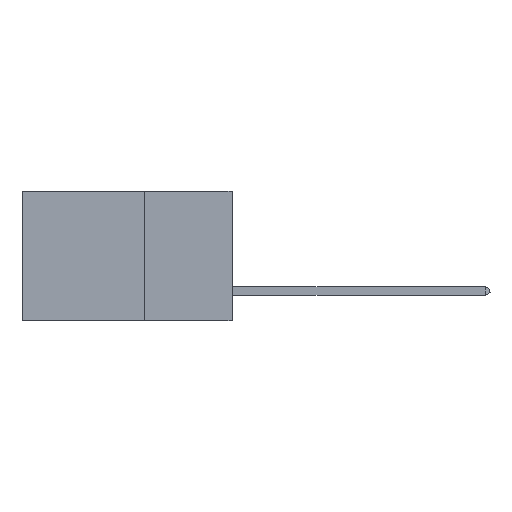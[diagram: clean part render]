
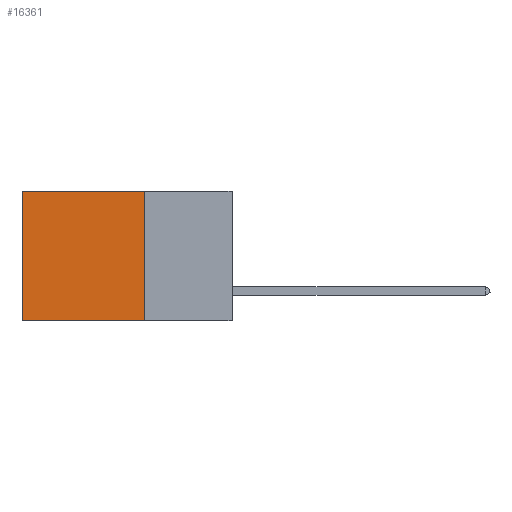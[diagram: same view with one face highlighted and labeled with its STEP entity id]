
A CAD part, left-side view. The second image highlights one B-rep face of the part: STEP entity #16361.
In plain terms, the highlighted planar face has unit normal (-1, 0, 0).
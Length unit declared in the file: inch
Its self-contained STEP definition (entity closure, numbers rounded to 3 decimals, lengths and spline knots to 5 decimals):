
#1655 = EDGE_LOOP ( 'NONE', ( #27776, #11221, #21335, #10406 ) ) ;
#3006 = VERTEX_POINT ( 'NONE', #31221 ) ;
#4205 = LINE ( 'NONE', #17229, #16119 ) ;
#4326 = LINE ( 'NONE', #5496, #10497 ) ;
#5043 = CARTESIAN_POINT ( 'NONE',  ( 0.2875, 0.25, 0. ) ) ;
#5496 = CARTESIAN_POINT ( 'NONE',  ( 0.2875, 0.25, 0. ) ) ;
#5628 = EDGE_CURVE ( 'NONE', #12628, #7341, #4205, .T. ) ;
#7341 = VERTEX_POINT ( 'NONE', #9530 ) ;
#7800 = DIRECTION ( 'NONE',  ( 0., 0., -1. ) ) ;
#9530 = CARTESIAN_POINT ( 'NONE',  ( 0.2875, 0.6, -0.37 ) ) ;
#9923 = CARTESIAN_POINT ( 'NONE',  ( 0.2875, 0.6, 0. ) ) ;
#10406 = ORIENTED_EDGE ( 'NONE', *, *, #24527, .T. ) ;
#10497 = VECTOR ( 'NONE', #31381, 39.37008 ) ;
#11221 = ORIENTED_EDGE ( 'NONE', *, *, #28537, .F. ) ;
#12135 = VECTOR ( 'NONE', #25882, 39.37008 ) ;
#12628 = VERTEX_POINT ( 'NONE', #9923 ) ;
#13090 = DIRECTION ( 'NONE',  ( 1., 0., 0. ) ) ;
#16119 = VECTOR ( 'NONE', #28268, 39.37008 ) ;
#16177 = LINE ( 'NONE', #26999, #20704 ) ;
#16361 = ADVANCED_FACE ( 'NONE', ( #22333 ), #20806, .F. ) ;
#17229 = CARTESIAN_POINT ( 'NONE',  ( 0.2875, 0.6, 0. ) ) ;
#17569 = AXIS2_PLACEMENT_3D ( 'NONE', #5043, #13090, #7800 ) ;
#20704 = VECTOR ( 'NONE', #32283, 39.37008 ) ;
#20806 = PLANE ( 'NONE',  #17569 ) ;
#20807 = LINE ( 'NONE', #25993, #12135 ) ;
#21335 = ORIENTED_EDGE ( 'NONE', *, *, #29887, .F. ) ;
#22022 = CARTESIAN_POINT ( 'NONE',  ( 0.2875, 0.25, 0. ) ) ;
#22333 = FACE_OUTER_BOUND ( 'NONE', #1655, .T. ) ;
#24527 = EDGE_CURVE ( 'NONE', #29879, #12628, #4326, .T. ) ;
#25882 = DIRECTION ( 'NONE',  ( 0., 1., 0. ) ) ;
#25993 = CARTESIAN_POINT ( 'NONE',  ( 0.2875, 0.25, -0.37 ) ) ;
#26999 = CARTESIAN_POINT ( 'NONE',  ( 0.2875, 0.25, 0. ) ) ;
#27776 = ORIENTED_EDGE ( 'NONE', *, *, #5628, .T. ) ;
#28268 = DIRECTION ( 'NONE',  ( 0., 0., -1. ) ) ;
#28537 = EDGE_CURVE ( 'NONE', #3006, #7341, #20807, .T. ) ;
#29879 = VERTEX_POINT ( 'NONE', #22022 ) ;
#29887 = EDGE_CURVE ( 'NONE', #29879, #3006, #16177, .T. ) ;
#31221 = CARTESIAN_POINT ( 'NONE',  ( 0.2875, 0.25, -0.37 ) ) ;
#31381 = DIRECTION ( 'NONE',  ( 0., 1., 0. ) ) ;
#32283 = DIRECTION ( 'NONE',  ( 0., 0., -1. ) ) ;
